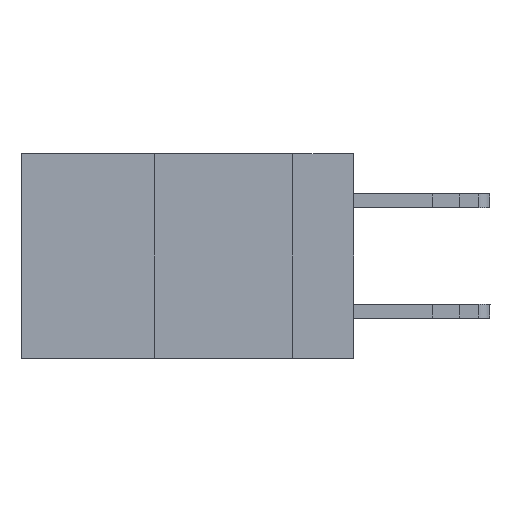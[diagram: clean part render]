
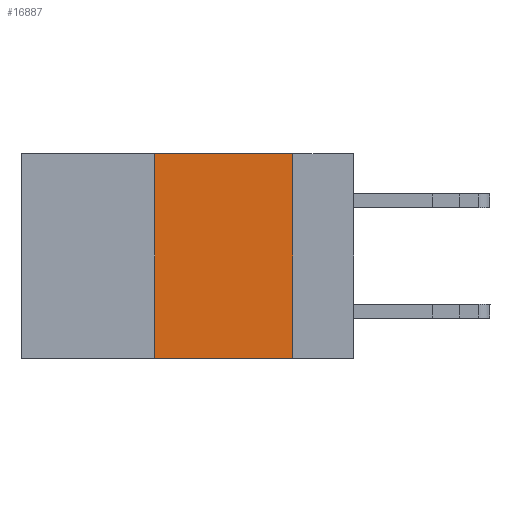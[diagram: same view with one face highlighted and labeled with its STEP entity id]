
A CAD part, left-side view. The second image highlights one B-rep face of the part: STEP entity #16887.
In plain terms, the highlighted planar face has unit normal (-1, 0, 0).
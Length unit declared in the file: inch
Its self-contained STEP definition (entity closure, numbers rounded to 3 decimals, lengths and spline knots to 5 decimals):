
#166 = DIRECTION ( 'NONE',  ( 0., -1., 0. ) ) ;
#605 = CARTESIAN_POINT ( 'NONE',  ( 0., 0.6, 0. ) ) ;
#789 = ORIENTED_EDGE ( 'NONE', *, *, #16005, .F. ) ;
#1123 = CARTESIAN_POINT ( 'NONE',  ( 0., 0.11, 0. ) ) ;
#1644 = VECTOR ( 'NONE', #17130, 39.37008 ) ;
#1889 = PLANE ( 'NONE',  #8953 ) ;
#1998 = EDGE_CURVE ( 'NONE', #17050, #3222, #14793, .T. ) ;
#2168 = EDGE_LOOP ( 'NONE', ( #789, #5516, #14892, #8851 ) ) ;
#2893 = VECTOR ( 'NONE', #166, 39.37008 ) ;
#3222 = VERTEX_POINT ( 'NONE', #14306 ) ;
#3385 = DIRECTION ( 'NONE',  ( 0., 0., -1. ) ) ;
#3586 = VERTEX_POINT ( 'NONE', #4558 ) ;
#4480 = VECTOR ( 'NONE', #6069, 39.37008 ) ;
#4558 = CARTESIAN_POINT ( 'NONE',  ( 0., 0.11, 0. ) ) ;
#5516 = ORIENTED_EDGE ( 'NONE', *, *, #15923, .F. ) ;
#5796 = CARTESIAN_POINT ( 'NONE',  ( 0., 0.6, -0.37 ) ) ;
#6069 = DIRECTION ( 'NONE',  ( 0., -1., 0. ) ) ;
#6347 = LINE ( 'NONE', #1123, #1644 ) ;
#7072 = CARTESIAN_POINT ( 'NONE',  ( 0., 0.36, -0.37 ) ) ;
#7078 = CARTESIAN_POINT ( 'NONE',  ( 0., 0.11, -0.37 ) ) ;
#7179 = DIRECTION ( 'NONE',  ( 0., 0., 1. ) ) ;
#7558 = EDGE_CURVE ( 'NONE', #17050, #14430, #12252, .T. ) ;
#8590 = CARTESIAN_POINT ( 'NONE',  ( 0., 0.6, 0. ) ) ;
#8851 = ORIENTED_EDGE ( 'NONE', *, *, #7558, .T. ) ;
#8953 = AXIS2_PLACEMENT_3D ( 'NONE', #8590, #10116, #3385 ) ;
#9812 = VECTOR ( 'NONE', #7179, 39.37008 ) ;
#10116 = DIRECTION ( 'NONE',  ( 1., 0., 0. ) ) ;
#10813 = CARTESIAN_POINT ( 'NONE',  ( 0., 0.36, 0. ) ) ;
#11250 = FACE_OUTER_BOUND ( 'NONE', #2168, .T. ) ;
#12252 = LINE ( 'NONE', #5796, #2893 ) ;
#14306 = CARTESIAN_POINT ( 'NONE',  ( 0., 0.36, 0. ) ) ;
#14430 = VERTEX_POINT ( 'NONE', #7078 ) ;
#14793 = LINE ( 'NONE', #10813, #9812 ) ;
#14892 = ORIENTED_EDGE ( 'NONE', *, *, #1998, .F. ) ;
#15161 = LINE ( 'NONE', #605, #4480 ) ;
#15923 = EDGE_CURVE ( 'NONE', #3222, #3586, #15161, .T. ) ;
#16005 = EDGE_CURVE ( 'NONE', #3586, #14430, #6347, .T. ) ;
#16887 = ADVANCED_FACE ( 'NONE', ( #11250 ), #1889, .F. ) ;
#17050 = VERTEX_POINT ( 'NONE', #7072 ) ;
#17130 = DIRECTION ( 'NONE',  ( 0., 0., -1. ) ) ;
